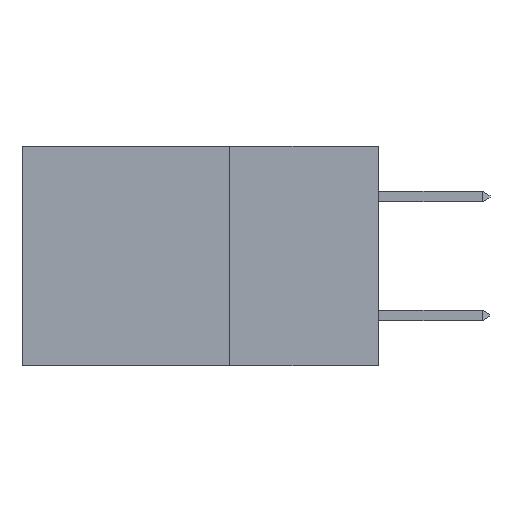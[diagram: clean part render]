
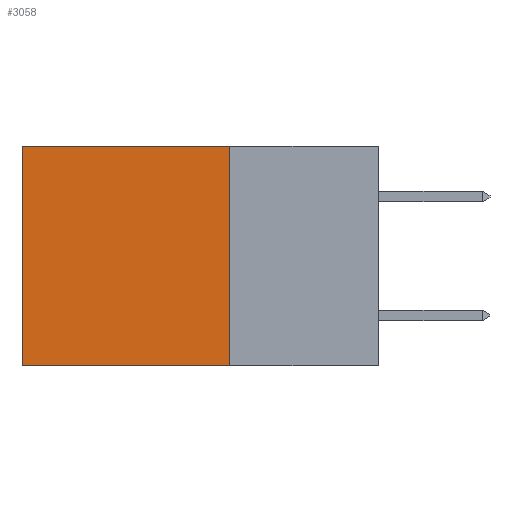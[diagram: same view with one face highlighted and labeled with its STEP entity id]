
A CAD part, left-side view. The second image highlights one B-rep face of the part: STEP entity #3058.
In plain terms, the highlighted planar face has unit normal (-1, 0, 0).
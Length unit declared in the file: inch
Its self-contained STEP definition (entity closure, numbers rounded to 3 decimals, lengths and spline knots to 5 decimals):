
#127 = ORIENTED_EDGE ( 'NONE', *, *, #3381, .F. ) ;
#181 = VERTEX_POINT ( 'NONE', #17941 ) ;
#232 = VECTOR ( 'NONE', #6894, 39.37008 ) ;
#2205 = PLANE ( 'NONE',  #2885 ) ;
#2285 = DIRECTION ( 'NONE',  ( 0., 1., 0. ) ) ;
#2574 = VECTOR ( 'NONE', #2285, 39.37008 ) ;
#2885 = AXIS2_PLACEMENT_3D ( 'NONE', #17241, #11801, #13311 ) ;
#2957 = FACE_OUTER_BOUND ( 'NONE', #3196, .T. ) ;
#3058 = ADVANCED_FACE ( 'NONE', ( #2957 ), #2205, .F. ) ;
#3196 = EDGE_LOOP ( 'NONE', ( #5915, #127, #11761, #12474 ) ) ;
#3381 = EDGE_CURVE ( 'NONE', #181, #8437, #12991, .T. ) ;
#3541 = DIRECTION ( 'NONE',  ( 0., 0., -1. ) ) ;
#5354 = CARTESIAN_POINT ( 'NONE',  ( 0.298, 0.25, 0. ) ) ;
#5915 = ORIENTED_EDGE ( 'NONE', *, *, #16944, .T. ) ;
#6068 = VECTOR ( 'NONE', #3541, 39.37008 ) ;
#6894 = DIRECTION ( 'NONE',  ( 0., 0., -1. ) ) ;
#8217 = VERTEX_POINT ( 'NONE', #19290 ) ;
#8437 = VERTEX_POINT ( 'NONE', #15258 ) ;
#8469 = VECTOR ( 'NONE', #15885, 39.37008 ) ;
#11156 = CARTESIAN_POINT ( 'NONE',  ( 0.298, 0.6, 0. ) ) ;
#11202 = EDGE_CURVE ( 'NONE', #15676, #8217, #18806, .T. ) ;
#11761 = ORIENTED_EDGE ( 'NONE', *, *, #14662, .F. ) ;
#11801 = DIRECTION ( 'NONE',  ( 1., 0., 0. ) ) ;
#12474 = ORIENTED_EDGE ( 'NONE', *, *, #11202, .T. ) ;
#12482 = LINE ( 'NONE', #5354, #232 ) ;
#12944 = CARTESIAN_POINT ( 'NONE',  ( 0.298, 0.25, -0.37 ) ) ;
#12991 = LINE ( 'NONE', #12944, #8469 ) ;
#13311 = DIRECTION ( 'NONE',  ( 0., 0., -1. ) ) ;
#14413 = CARTESIAN_POINT ( 'NONE',  ( 0.298, 0.25, 0. ) ) ;
#14662 = EDGE_CURVE ( 'NONE', #15676, #181, #12482, .T. ) ;
#15258 = CARTESIAN_POINT ( 'NONE',  ( 0.298, 0.6, -0.37 ) ) ;
#15676 = VERTEX_POINT ( 'NONE', #18990 ) ;
#15885 = DIRECTION ( 'NONE',  ( 0., 1., 0. ) ) ;
#16944 = EDGE_CURVE ( 'NONE', #8217, #8437, #18215, .T. ) ;
#17241 = CARTESIAN_POINT ( 'NONE',  ( 0.298, 0.25, 0. ) ) ;
#17941 = CARTESIAN_POINT ( 'NONE',  ( 0.298, 0.25, -0.37 ) ) ;
#18215 = LINE ( 'NONE', #11156, #6068 ) ;
#18806 = LINE ( 'NONE', #14413, #2574 ) ;
#18990 = CARTESIAN_POINT ( 'NONE',  ( 0.298, 0.25, 0. ) ) ;
#19290 = CARTESIAN_POINT ( 'NONE',  ( 0.298, 0.6, 0. ) ) ;
